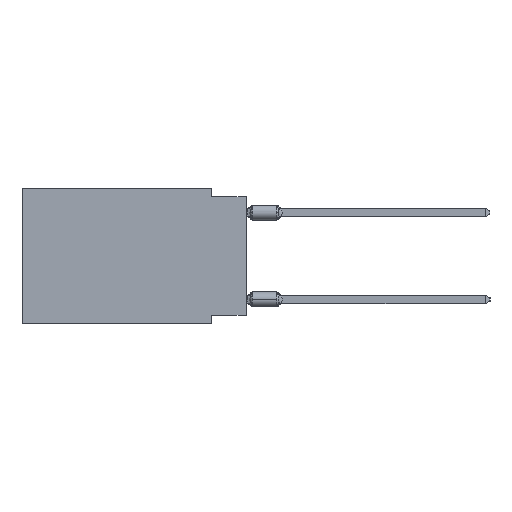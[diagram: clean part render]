
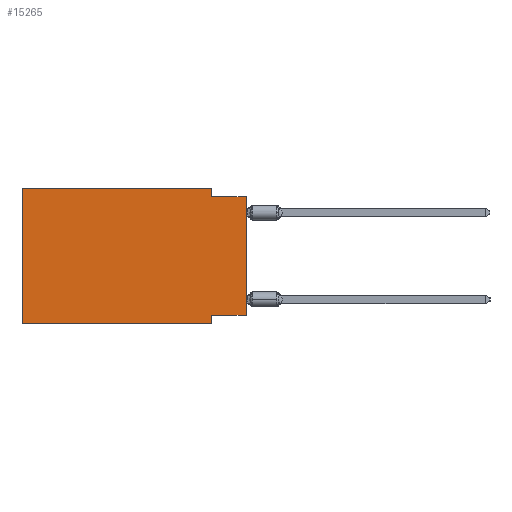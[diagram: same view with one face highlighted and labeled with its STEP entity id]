
A CAD part, left-side view. The second image highlights one B-rep face of the part: STEP entity #15265.
In plain terms, the highlighted planar face has unit normal (-1, 0, 0).
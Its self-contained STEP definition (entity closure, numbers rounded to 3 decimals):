
#2333 = ORIENTED_EDGE ( 'NONE', *, *, #24381, .F. ) ;
#2537 = DIRECTION ( 'NONE',  ( 0., 1., 0. ) ) ;
#4302 = DIRECTION ( 'NONE',  ( 1., 0., 0. ) ) ;
#4424 = CARTESIAN_POINT ( 'NONE',  ( 0., 2.54, -9.271 ) ) ;
#5476 = CARTESIAN_POINT ( 'NONE',  ( 0., 16.383, 0. ) ) ;
#6587 = VERTEX_POINT ( 'NONE', #24308 ) ;
#8282 = EDGE_CURVE ( 'NONE', #6587, #29924, #15745, .T. ) ;
#9257 = VERTEX_POINT ( 'NONE', #47770 ) ;
#9418 = EDGE_CURVE ( 'NONE', #37253, #47834, #44546, .T. ) ;
#9579 = EDGE_CURVE ( 'NONE', #29924, #30862, #49690, .T. ) ;
#10614 = ORIENTED_EDGE ( 'NONE', *, *, #9418, .F. ) ;
#13370 = LINE ( 'NONE', #17482, #52178 ) ;
#14085 = DIRECTION ( 'NONE',  ( 0., -1., 0. ) ) ;
#15265 = ADVANCED_FACE ( 'NONE', ( #26556 ), #34748, .F. ) ;
#15745 = LINE ( 'NONE', #29210, #55873 ) ;
#15884 = ORIENTED_EDGE ( 'NONE', *, *, #34389, .T. ) ;
#15975 = ORIENTED_EDGE ( 'NONE', *, *, #46436, .F. ) ;
#15979 = CARTESIAN_POINT ( 'NONE',  ( 0., 2.54, 0. ) ) ;
#17482 = CARTESIAN_POINT ( 'NONE',  ( 0., 2.54, -9.906 ) ) ;
#17582 = VECTOR ( 'NONE', #19533, 1000. ) ;
#17675 = VECTOR ( 'NONE', #14085, 1000. ) ;
#19533 = DIRECTION ( 'NONE',  ( 0., -1., 0. ) ) ;
#24308 = CARTESIAN_POINT ( 'NONE',  ( 0., 16.383, -9.906 ) ) ;
#24381 = EDGE_CURVE ( 'NONE', #48700, #9257, #13370, .T. ) ;
#24769 = CARTESIAN_POINT ( 'NONE',  ( 0., 0., -9.271 ) ) ;
#25984 = DIRECTION ( 'NONE',  ( 0., 0., -1. ) ) ;
#26271 = VECTOR ( 'NONE', #45600, 1000. ) ;
#26556 = FACE_OUTER_BOUND ( 'NONE', #28634, .T. ) ;
#26749 = CARTESIAN_POINT ( 'NONE',  ( 0., 0., 0. ) ) ;
#28164 = CARTESIAN_POINT ( 'NONE',  ( 0., 2.54, 0. ) ) ;
#28634 = EDGE_LOOP ( 'NONE', ( #15884, #10614, #30244, #28709, #38308, #57174, #2333, #15975 ) ) ;
#28709 = ORIENTED_EDGE ( 'NONE', *, *, #9579, .F. ) ;
#29210 = CARTESIAN_POINT ( 'NONE',  ( 0., 16.383, 0. ) ) ;
#29924 = VERTEX_POINT ( 'NONE', #5476 ) ;
#30044 = AXIS2_PLACEMENT_3D ( 'NONE', #52586, #4302, #57263 ) ;
#30244 = ORIENTED_EDGE ( 'NONE', *, *, #52133, .F. ) ;
#30328 = LINE ( 'NONE', #24769, #30708 ) ;
#30708 = VECTOR ( 'NONE', #2537, 1000. ) ;
#30862 = VERTEX_POINT ( 'NONE', #28164 ) ;
#32413 = CARTESIAN_POINT ( 'NONE',  ( 0., 16.383, -9.906 ) ) ;
#32998 = CARTESIAN_POINT ( 'NONE',  ( 0., 0., -9.271 ) ) ;
#33683 = VERTEX_POINT ( 'NONE', #32998 ) ;
#34389 = EDGE_CURVE ( 'NONE', #33683, #47834, #36403, .T. ) ;
#34501 = CARTESIAN_POINT ( 'NONE',  ( 0., 0., -0.635 ) ) ;
#34748 = PLANE ( 'NONE',  #30044 ) ;
#36403 = LINE ( 'NONE', #26749, #55726 ) ;
#37253 = VERTEX_POINT ( 'NONE', #45847 ) ;
#38308 = ORIENTED_EDGE ( 'NONE', *, *, #8282, .F. ) ;
#40182 = CARTESIAN_POINT ( 'NONE',  ( 0., 0., -0.635 ) ) ;
#40647 = CARTESIAN_POINT ( 'NONE',  ( 0., 16.383, 0. ) ) ;
#40792 = DIRECTION ( 'NONE',  ( 0., 0., 1. ) ) ;
#42285 = VECTOR ( 'NONE', #56064, 1000. ) ;
#42918 = LINE ( 'NONE', #15979, #42285 ) ;
#44546 = LINE ( 'NONE', #40182, #17675 ) ;
#44675 = EDGE_CURVE ( 'NONE', #6587, #9257, #50249, .T. ) ;
#45600 = DIRECTION ( 'NONE',  ( 0., -1., 0. ) ) ;
#45847 = CARTESIAN_POINT ( 'NONE',  ( 0., 2.54, -0.635 ) ) ;
#46436 = EDGE_CURVE ( 'NONE', #33683, #48700, #30328, .T. ) ;
#47770 = CARTESIAN_POINT ( 'NONE',  ( 0., 2.54, -9.906 ) ) ;
#47834 = VERTEX_POINT ( 'NONE', #34501 ) ;
#48700 = VERTEX_POINT ( 'NONE', #4424 ) ;
#49690 = LINE ( 'NONE', #40647, #26271 ) ;
#50249 = LINE ( 'NONE', #32413, #17582 ) ;
#52133 = EDGE_CURVE ( 'NONE', #30862, #37253, #42918, .T. ) ;
#52178 = VECTOR ( 'NONE', #25984, 1000. ) ;
#52586 = CARTESIAN_POINT ( 'NONE',  ( 0., 16.383, 0. ) ) ;
#54962 = DIRECTION ( 'NONE',  ( 0., 0., 1. ) ) ;
#55726 = VECTOR ( 'NONE', #40792, 1000. ) ;
#55873 = VECTOR ( 'NONE', #54962, 1000. ) ;
#56064 = DIRECTION ( 'NONE',  ( 0., 0., -1. ) ) ;
#57174 = ORIENTED_EDGE ( 'NONE', *, *, #44675, .T. ) ;
#57263 = DIRECTION ( 'NONE',  ( 0., 0., -1. ) ) ;
